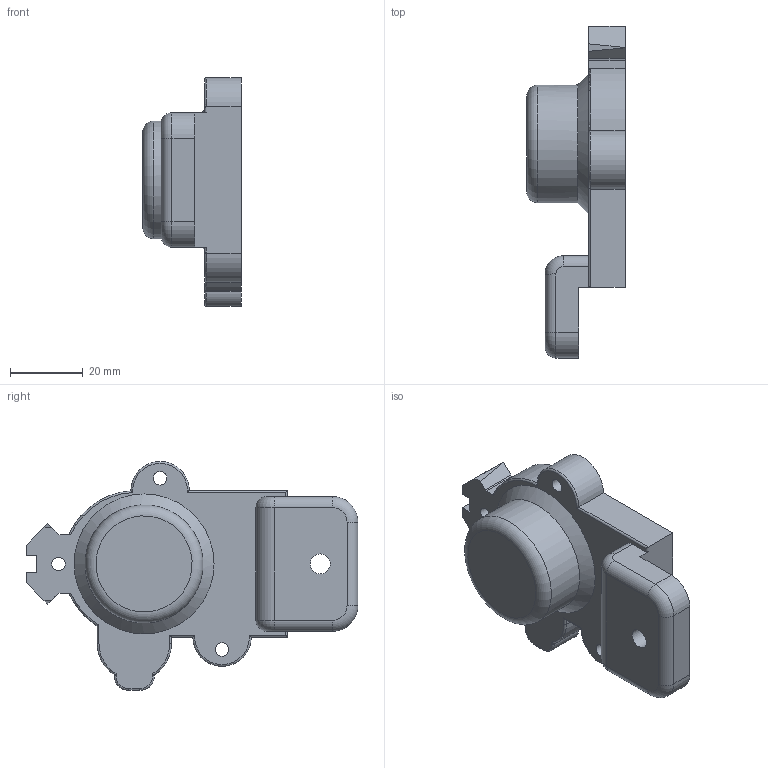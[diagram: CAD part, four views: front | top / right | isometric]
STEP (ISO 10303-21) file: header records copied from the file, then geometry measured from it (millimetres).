
FILE_DESCRIPTION (( 'STEP AP203' ), '1' );
FILE_NAME ('WTF-9_hillbilly_endcap.STEP', '2020-05-09T08:51:08', ( '' ), ( '' ), 'SwSTEP 2.0', 'SolidWorks 2016', '' );
FILE_SCHEMA (( 'CONFIG_CONTROL_DESIGN' ));
Length unit declared in the file: millimetre
Products named in the file (2): WTF HILLBILLY FINAL_5; WTF-9_hillbilly_endcap
Assembly tree (1 placements, depth 2):
  WTF-9_hillbilly_endcap
    WTF HILLBILLY FINAL_5
Bounding box: 27 x 91.08 x 62.82 mm (x, y, z)
Volume: 43660 mm3; surface area: 14262 mm2
Topology: 1 solids, 1 shells, 81 faces, 207 edges, 130 vertices
Faces by surface type: plane 34, cylinder 32, torus 13, cone 2
Full cylindrical faces by diameter (mm): 3.7 x3, 5.5 x1, 22.8 x1, 32.4 x1
Entity records: 2669 total; most frequent: CARTESIAN_POINT 519, DIRECTION 422, ORIENTED_EDGE 392, EDGE_CURVE 196, AXIS2_PLACEMENT_3D 153, VERTEX_POINT 128, LINE 116, VECTOR 116
